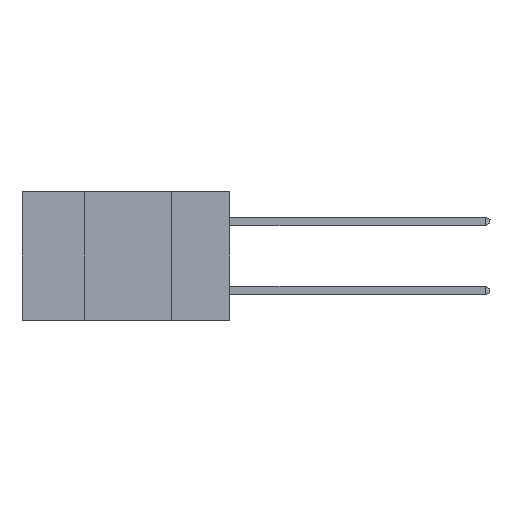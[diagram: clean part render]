
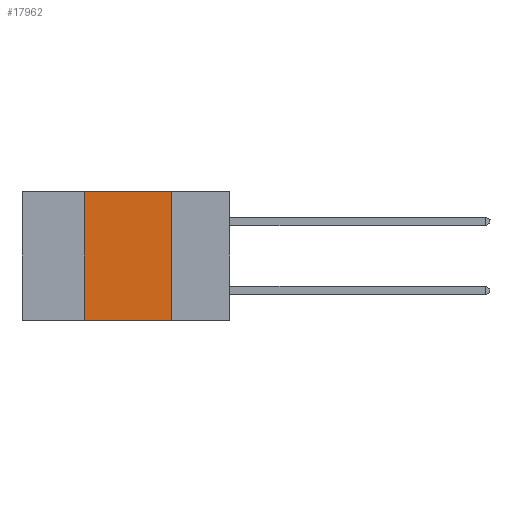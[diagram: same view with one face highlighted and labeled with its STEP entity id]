
A CAD part, left-side view. The second image highlights one B-rep face of the part: STEP entity #17962.
In plain terms, the highlighted planar face has unit normal (-1, 0, 0).
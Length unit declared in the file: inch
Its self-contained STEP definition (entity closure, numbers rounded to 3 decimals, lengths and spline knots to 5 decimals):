
#265 = DIRECTION ( 'NONE',  ( 0., 0., -1. ) ) ;
#531 = CARTESIAN_POINT ( 'NONE',  ( 0., 0.42, 0. ) ) ;
#705 = CARTESIAN_POINT ( 'NONE',  ( 0., 0.42, -0.37 ) ) ;
#1450 = CARTESIAN_POINT ( 'NONE',  ( 0., 0.6, -0.37 ) ) ;
#1798 = EDGE_CURVE ( 'NONE', #2272, #5080, #2015, .T. ) ;
#2015 = LINE ( 'NONE', #18017, #6806 ) ;
#2105 = DIRECTION ( 'NONE',  ( 0., -1., 0. ) ) ;
#2272 = VERTEX_POINT ( 'NONE', #531 ) ;
#3001 = EDGE_CURVE ( 'NONE', #5080, #15564, #9775, .T. ) ;
#5047 = DIRECTION ( 'NONE',  ( 1., 0., 0. ) ) ;
#5080 = VERTEX_POINT ( 'NONE', #15094 ) ;
#5864 = LINE ( 'NONE', #1450, #9742 ) ;
#5886 = EDGE_CURVE ( 'NONE', #12262, #15564, #5864, .T. ) ;
#6119 = PLANE ( 'NONE',  #13752 ) ;
#6806 = VECTOR ( 'NONE', #2105, 39.37008 ) ;
#7195 = EDGE_LOOP ( 'NONE', ( #13685, #14548, #9594, #7202 ) ) ;
#7202 = ORIENTED_EDGE ( 'NONE', *, *, #5886, .T. ) ;
#8567 = VECTOR ( 'NONE', #17106, 39.37008 ) ;
#9585 = DIRECTION ( 'NONE',  ( 0., 0., -1. ) ) ;
#9594 = ORIENTED_EDGE ( 'NONE', *, *, #18484, .F. ) ;
#9742 = VECTOR ( 'NONE', #11701, 39.37008 ) ;
#9775 = LINE ( 'NONE', #14062, #17268 ) ;
#10465 = CARTESIAN_POINT ( 'NONE',  ( 0., 0.42, -0.37 ) ) ;
#11701 = DIRECTION ( 'NONE',  ( 0., -1., 0. ) ) ;
#12262 = VERTEX_POINT ( 'NONE', #10465 ) ;
#12328 = FACE_OUTER_BOUND ( 'NONE', #7195, .T. ) ;
#13685 = ORIENTED_EDGE ( 'NONE', *, *, #3001, .F. ) ;
#13752 = AXIS2_PLACEMENT_3D ( 'NONE', #18186, #5047, #265 ) ;
#14062 = CARTESIAN_POINT ( 'NONE',  ( 0., 0.17, -0.37 ) ) ;
#14548 = ORIENTED_EDGE ( 'NONE', *, *, #1798, .F. ) ;
#15094 = CARTESIAN_POINT ( 'NONE',  ( 0., 0.17, 0. ) ) ;
#15564 = VERTEX_POINT ( 'NONE', #18580 ) ;
#16722 = LINE ( 'NONE', #705, #8567 ) ;
#17106 = DIRECTION ( 'NONE',  ( 0., 0., 1. ) ) ;
#17268 = VECTOR ( 'NONE', #9585, 39.37008 ) ;
#17962 = ADVANCED_FACE ( 'NONE', ( #12328 ), #6119, .F. ) ;
#18017 = CARTESIAN_POINT ( 'NONE',  ( 0., 0.6, 0. ) ) ;
#18186 = CARTESIAN_POINT ( 'NONE',  ( 0., 0.6, 0. ) ) ;
#18484 = EDGE_CURVE ( 'NONE', #12262, #2272, #16722, .T. ) ;
#18580 = CARTESIAN_POINT ( 'NONE',  ( 0., 0.17, -0.37 ) ) ;
